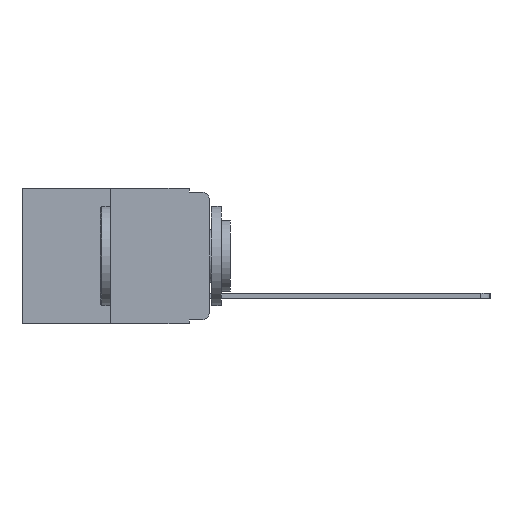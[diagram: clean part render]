
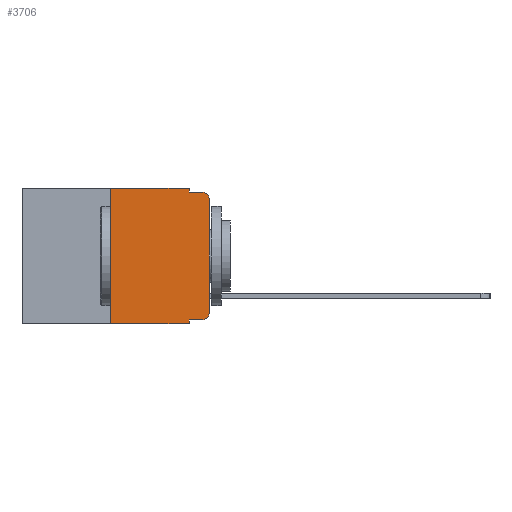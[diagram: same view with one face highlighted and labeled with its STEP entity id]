
A CAD part, left-side view. The second image highlights one B-rep face of the part: STEP entity #3706.
In plain terms, the highlighted planar face has unit normal (-1, 0, 0).
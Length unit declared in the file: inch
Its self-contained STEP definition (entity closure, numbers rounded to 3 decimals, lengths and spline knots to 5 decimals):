
#551 = ORIENTED_EDGE ( 'NONE', *, *, #855, .F. ) ;
#602 = VERTEX_POINT ( 'NONE', #10704 ) ;
#855 = EDGE_CURVE ( 'NONE', #602, #6465, #10921, .T. ) ;
#1278 = LINE ( 'NONE', #1751, #7968 ) ;
#1751 = CARTESIAN_POINT ( 'NONE',  ( 0., 0.25, 0. ) ) ;
#1769 = EDGE_CURVE ( 'NONE', #6465, #9788, #4325, .T. ) ;
#1951 = EDGE_LOOP ( 'NONE', ( #14791, #6646, #14236, #6044, #551, #9562, #11429, #8975, #12887, #10505 ) ) ;
#2048 = VERTEX_POINT ( 'NONE', #11142 ) ;
#2097 = AXIS2_PLACEMENT_3D ( 'NONE', #13445, #2133, #11131 ) ;
#2133 = DIRECTION ( 'NONE',  ( 1., 0., 0. ) ) ;
#2348 = CARTESIAN_POINT ( 'NONE',  ( 0., 0.02, -0.333 ) ) ;
#2814 = VECTOR ( 'NONE', #12877, 39.37008 ) ;
#2842 = VERTEX_POINT ( 'NONE', #9271 ) ;
#3251 = LINE ( 'NONE', #7789, #15657 ) ;
#3490 = CARTESIAN_POINT ( 'NONE',  ( 0., 0.051, -0.343 ) ) ;
#3616 = LINE ( 'NONE', #13413, #10073 ) ;
#3706 = ADVANCED_FACE ( 'NONE', ( #15858 ), #9936, .F. ) ;
#3806 = CARTESIAN_POINT ( 'NONE',  ( 0., 0.051, 0. ) ) ;
#4036 = CARTESIAN_POINT ( 'NONE',  ( 0., 0.02, -0.03 ) ) ;
#4325 = LINE ( 'NONE', #3806, #7411 ) ;
#5318 = CIRCLE ( 'NONE', #12910, 0.02 ) ;
#5391 = DIRECTION ( 'NONE',  ( 0., 0., -1. ) ) ;
#5506 = EDGE_CURVE ( 'NONE', #2842, #8427, #12266, .T. ) ;
#5550 = CARTESIAN_POINT ( 'NONE',  ( 0., 0.25, -0.343 ) ) ;
#5849 = EDGE_CURVE ( 'NONE', #14879, #2048, #10823, .T. ) ;
#5865 = EDGE_CURVE ( 'NONE', #2048, #11252, #3616, .T. ) ;
#5928 = CARTESIAN_POINT ( 'NONE',  ( 0., 0.051, -0.01 ) ) ;
#6044 = ORIENTED_EDGE ( 'NONE', *, *, #1769, .F. ) ;
#6465 = VERTEX_POINT ( 'NONE', #9945 ) ;
#6646 = ORIENTED_EDGE ( 'NONE', *, *, #13565, .T. ) ;
#6755 = CARTESIAN_POINT ( 'NONE',  ( 0., 0.051, -0.333 ) ) ;
#6986 = CARTESIAN_POINT ( 'NONE',  ( 0., 0.473, -0.343 ) ) ;
#7178 = VERTEX_POINT ( 'NONE', #13540 ) ;
#7340 = DIRECTION ( 'NONE',  ( -1., 0., 0. ) ) ;
#7411 = VECTOR ( 'NONE', #11406, 39.37008 ) ;
#7647 = VECTOR ( 'NONE', #13870, 39.37008 ) ;
#7675 = CARTESIAN_POINT ( 'NONE',  ( 0., 0.02, -0.313 ) ) ;
#7789 = CARTESIAN_POINT ( 'NONE',  ( 0., 0.051, -0.01 ) ) ;
#7943 = CARTESIAN_POINT ( 'NONE',  ( 0., 0.473, 0. ) ) ;
#7968 = VECTOR ( 'NONE', #13185, 39.37008 ) ;
#8145 = VERTEX_POINT ( 'NONE', #5550 ) ;
#8274 = DIRECTION ( 'NONE',  ( 0., -1., 0. ) ) ;
#8427 = VERTEX_POINT ( 'NONE', #3490 ) ;
#8975 = ORIENTED_EDGE ( 'NONE', *, *, #5506, .F. ) ;
#9042 = DIRECTION ( 'NONE',  ( 0., -1., 0. ) ) ;
#9101 = VECTOR ( 'NONE', #16229, 39.37008 ) ;
#9271 = CARTESIAN_POINT ( 'NONE',  ( 0., 0.051, -0.333 ) ) ;
#9562 = ORIENTED_EDGE ( 'NONE', *, *, #15814, .F. ) ;
#9788 = VERTEX_POINT ( 'NONE', #5928 ) ;
#9848 = CARTESIAN_POINT ( 'NONE',  ( 0., 0., -0.03 ) ) ;
#9936 = PLANE ( 'NONE',  #2097 ) ;
#9945 = CARTESIAN_POINT ( 'NONE',  ( 0., 0.051, 0. ) ) ;
#10073 = VECTOR ( 'NONE', #14592, 39.37008 ) ;
#10505 = ORIENTED_EDGE ( 'NONE', *, *, #5849, .T. ) ;
#10704 = CARTESIAN_POINT ( 'NONE',  ( 0., 0.25, 0. ) ) ;
#10823 = CIRCLE ( 'NONE', #13861, 0.02 ) ;
#10921 = LINE ( 'NONE', #7943, #7647 ) ;
#11131 = DIRECTION ( 'NONE',  ( 0., 0., -1. ) ) ;
#11142 = CARTESIAN_POINT ( 'NONE',  ( 0., 0., -0.313 ) ) ;
#11252 = VERTEX_POINT ( 'NONE', #9848 ) ;
#11406 = DIRECTION ( 'NONE',  ( 0., 0., -1. ) ) ;
#11429 = ORIENTED_EDGE ( 'NONE', *, *, #11568, .T. ) ;
#11568 = EDGE_CURVE ( 'NONE', #8145, #8427, #13649, .T. ) ;
#12266 = LINE ( 'NONE', #12658, #9101 ) ;
#12658 = CARTESIAN_POINT ( 'NONE',  ( 0., 0.051, 0. ) ) ;
#12773 = DIRECTION ( 'NONE',  ( -1., 0., 0. ) ) ;
#12860 = LINE ( 'NONE', #6755, #2814 ) ;
#12877 = DIRECTION ( 'NONE',  ( 0., -1., 0. ) ) ;
#12887 = ORIENTED_EDGE ( 'NONE', *, *, #13242, .T. ) ;
#12910 = AXIS2_PLACEMENT_3D ( 'NONE', #4036, #12773, #5391 ) ;
#13185 = DIRECTION ( 'NONE',  ( 0., 0., 1. ) ) ;
#13242 = EDGE_CURVE ( 'NONE', #2842, #14879, #12860, .T. ) ;
#13275 = VECTOR ( 'NONE', #8274, 39.37008 ) ;
#13413 = CARTESIAN_POINT ( 'NONE',  ( 0., 0., 0. ) ) ;
#13445 = CARTESIAN_POINT ( 'NONE',  ( 0., 0.473, 0. ) ) ;
#13540 = CARTESIAN_POINT ( 'NONE',  ( 0., 0.02, -0.01 ) ) ;
#13565 = EDGE_CURVE ( 'NONE', #11252, #7178, #5318, .T. ) ;
#13649 = LINE ( 'NONE', #6986, #13275 ) ;
#13861 = AXIS2_PLACEMENT_3D ( 'NONE', #7675, #7340, #15733 ) ;
#13870 = DIRECTION ( 'NONE',  ( 0., -1., 0. ) ) ;
#14236 = ORIENTED_EDGE ( 'NONE', *, *, #14941, .F. ) ;
#14592 = DIRECTION ( 'NONE',  ( 0., 0., 1. ) ) ;
#14791 = ORIENTED_EDGE ( 'NONE', *, *, #5865, .T. ) ;
#14879 = VERTEX_POINT ( 'NONE', #2348 ) ;
#14941 = EDGE_CURVE ( 'NONE', #9788, #7178, #3251, .T. ) ;
#15657 = VECTOR ( 'NONE', #9042, 39.37008 ) ;
#15733 = DIRECTION ( 'NONE',  ( 0., 0., -1. ) ) ;
#15814 = EDGE_CURVE ( 'NONE', #8145, #602, #1278, .T. ) ;
#15858 = FACE_OUTER_BOUND ( 'NONE', #1951, .T. ) ;
#16229 = DIRECTION ( 'NONE',  ( 0., 0., -1. ) ) ;
